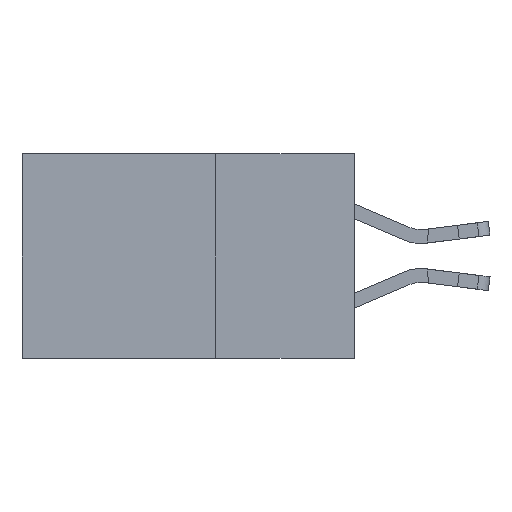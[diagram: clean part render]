
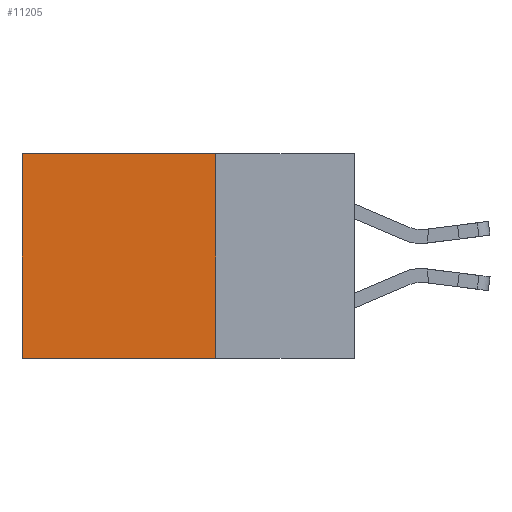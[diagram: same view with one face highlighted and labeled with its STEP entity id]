
A CAD part, left-side view. The second image highlights one B-rep face of the part: STEP entity #11205.
In plain terms, the highlighted planar face has unit normal (-1, 0, 0).
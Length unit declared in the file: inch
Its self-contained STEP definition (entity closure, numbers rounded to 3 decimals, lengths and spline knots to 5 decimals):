
#291 = CARTESIAN_POINT ( 'NONE',  ( 0.2615, 0.6, 0. ) ) ;
#452 = LINE ( 'NONE', #13114, #12594 ) ;
#666 = VECTOR ( 'NONE', #7736, 39.37008 ) ;
#1795 = VECTOR ( 'NONE', #11793, 39.37008 ) ;
#3450 = ORIENTED_EDGE ( 'NONE', *, *, #10219, .T. ) ;
#4021 = AXIS2_PLACEMENT_3D ( 'NONE', #7037, #7021, #7001 ) ;
#4354 = EDGE_CURVE ( 'NONE', #11946, #8382, #452, .T. ) ;
#5497 = FACE_OUTER_BOUND ( 'NONE', #8797, .T. ) ;
#5579 = CARTESIAN_POINT ( 'NONE',  ( 0.2615, 0.6, -0.37 ) ) ;
#5692 = CARTESIAN_POINT ( 'NONE',  ( 0.2615, 0.25, -0.37 ) ) ;
#7001 = DIRECTION ( 'NONE',  ( 0., 0., -1. ) ) ;
#7021 = DIRECTION ( 'NONE',  ( 1., 0., 0. ) ) ;
#7037 = CARTESIAN_POINT ( 'NONE',  ( 0.2615, 0.25, -0.37 ) ) ;
#7072 = PLANE ( 'NONE',  #4021 ) ;
#7279 = CARTESIAN_POINT ( 'NONE',  ( 0.2615, 0.25, 0. ) ) ;
#7655 = CARTESIAN_POINT ( 'NONE',  ( 0.2615, 0.25, -0.37 ) ) ;
#7736 = DIRECTION ( 'NONE',  ( 0., 0., -1. ) ) ;
#8091 = EDGE_CURVE ( 'NONE', #8165, #9891, #13145, .T. ) ;
#8165 = VERTEX_POINT ( 'NONE', #7279 ) ;
#8272 = LINE ( 'NONE', #14180, #11677 ) ;
#8382 = VERTEX_POINT ( 'NONE', #5579 ) ;
#8435 = LINE ( 'NONE', #11982, #1795 ) ;
#8797 = EDGE_LOOP ( 'NONE', ( #11968, #9253, #12302, #3450 ) ) ;
#9253 = ORIENTED_EDGE ( 'NONE', *, *, #10501, .F. ) ;
#9891 = VERTEX_POINT ( 'NONE', #5692 ) ;
#10219 = EDGE_CURVE ( 'NONE', #8165, #11946, #8272, .T. ) ;
#10501 = EDGE_CURVE ( 'NONE', #9891, #8382, #8435, .T. ) ;
#11205 = ADVANCED_FACE ( 'NONE', ( #5497 ), #7072, .F. ) ;
#11677 = VECTOR ( 'NONE', #14262, 39.37008 ) ;
#11793 = DIRECTION ( 'NONE',  ( 0., 1., 0. ) ) ;
#11946 = VERTEX_POINT ( 'NONE', #291 ) ;
#11968 = ORIENTED_EDGE ( 'NONE', *, *, #4354, .T. ) ;
#11982 = CARTESIAN_POINT ( 'NONE',  ( 0.2615, 0.25, -0.37 ) ) ;
#12302 = ORIENTED_EDGE ( 'NONE', *, *, #8091, .F. ) ;
#12594 = VECTOR ( 'NONE', #12885, 39.37008 ) ;
#12885 = DIRECTION ( 'NONE',  ( 0., 0., -1. ) ) ;
#13114 = CARTESIAN_POINT ( 'NONE',  ( 0.2615, 0.6, -0.37 ) ) ;
#13145 = LINE ( 'NONE', #7655, #666 ) ;
#14180 = CARTESIAN_POINT ( 'NONE',  ( 0.2615, 0.25, 0. ) ) ;
#14262 = DIRECTION ( 'NONE',  ( 0., 1., 0. ) ) ;
